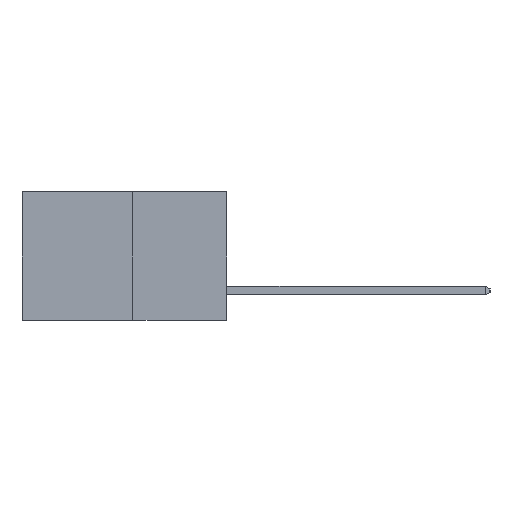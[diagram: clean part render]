
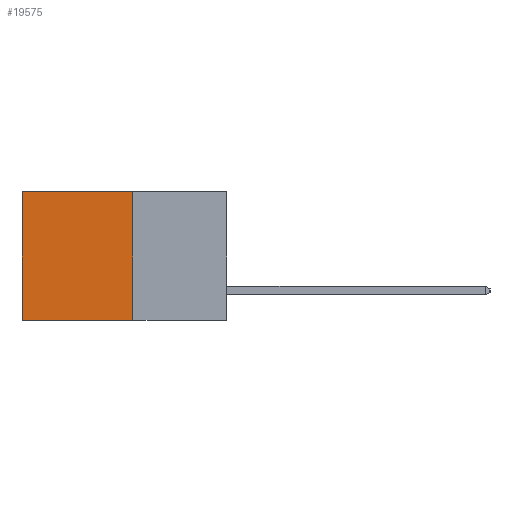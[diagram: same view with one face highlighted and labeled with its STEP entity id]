
A CAD part, left-side view. The second image highlights one B-rep face of the part: STEP entity #19575.
In plain terms, the highlighted planar face has unit normal (-1, 0, 0).
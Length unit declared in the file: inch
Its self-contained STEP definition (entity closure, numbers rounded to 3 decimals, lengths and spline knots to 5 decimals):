
#39 = DIRECTION ( 'NONE',  ( 1., 0., 0. ) ) ;
#659 = DIRECTION ( 'NONE',  ( 0., 1., 0. ) ) ;
#2499 = ORIENTED_EDGE ( 'NONE', *, *, #3594, .T. ) ;
#3594 = EDGE_CURVE ( 'NONE', #18828, #7540, #14032, .T. ) ;
#4113 = CARTESIAN_POINT ( 'NONE',  ( 0.277, 0.59, 0. ) ) ;
#4185 = EDGE_LOOP ( 'NONE', ( #10382, #17021, #5811, #2499 ) ) ;
#4565 = VECTOR ( 'NONE', #659, 39.37008 ) ;
#4894 = LINE ( 'NONE', #9921, #16411 ) ;
#5293 = FACE_OUTER_BOUND ( 'NONE', #4185, .T. ) ;
#5576 = CARTESIAN_POINT ( 'NONE',  ( 0.277, 0.27, 0. ) ) ;
#5670 = DIRECTION ( 'NONE',  ( 0., 1., 0. ) ) ;
#5811 = ORIENTED_EDGE ( 'NONE', *, *, #25685, .F. ) ;
#7540 = VERTEX_POINT ( 'NONE', #4113 ) ;
#8253 = VECTOR ( 'NONE', #5670, 39.37008 ) ;
#8951 = AXIS2_PLACEMENT_3D ( 'NONE', #10839, #39, #15227 ) ;
#9921 = CARTESIAN_POINT ( 'NONE',  ( 0.277, 0.27, -0.37 ) ) ;
#10382 = ORIENTED_EDGE ( 'NONE', *, *, #23854, .T. ) ;
#10839 = CARTESIAN_POINT ( 'NONE',  ( 0.277, 0.27, -0.37 ) ) ;
#12262 = CARTESIAN_POINT ( 'NONE',  ( 0.277, 0.27, 0. ) ) ;
#14032 = LINE ( 'NONE', #5576, #8253 ) ;
#15227 = DIRECTION ( 'NONE',  ( 0., 0., -1. ) ) ;
#15447 = LINE ( 'NONE', #15829, #4565 ) ;
#15829 = CARTESIAN_POINT ( 'NONE',  ( 0.277, 0.27, -0.37 ) ) ;
#16411 = VECTOR ( 'NONE', #25061, 39.37008 ) ;
#16643 = DIRECTION ( 'NONE',  ( 0., 0., -1. ) ) ;
#17021 = ORIENTED_EDGE ( 'NONE', *, *, #25526, .F. ) ;
#18231 = CARTESIAN_POINT ( 'NONE',  ( 0.277, 0.27, -0.37 ) ) ;
#18828 = VERTEX_POINT ( 'NONE', #12262 ) ;
#19575 = ADVANCED_FACE ( 'NONE', ( #5293 ), #25965, .F. ) ;
#21113 = CARTESIAN_POINT ( 'NONE',  ( 0.277, 0.59, -0.37 ) ) ;
#21858 = VERTEX_POINT ( 'NONE', #18231 ) ;
#23854 = EDGE_CURVE ( 'NONE', #7540, #25840, #27711, .T. ) ;
#25061 = DIRECTION ( 'NONE',  ( 0., 0., -1. ) ) ;
#25526 = EDGE_CURVE ( 'NONE', #21858, #25840, #15447, .T. ) ;
#25685 = EDGE_CURVE ( 'NONE', #18828, #21858, #4894, .T. ) ;
#25840 = VERTEX_POINT ( 'NONE', #21113 ) ;
#25965 = PLANE ( 'NONE',  #8951 ) ;
#27032 = VECTOR ( 'NONE', #16643, 39.37008 ) ;
#27386 = CARTESIAN_POINT ( 'NONE',  ( 0.277, 0.59, -0.37 ) ) ;
#27711 = LINE ( 'NONE', #27386, #27032 ) ;
